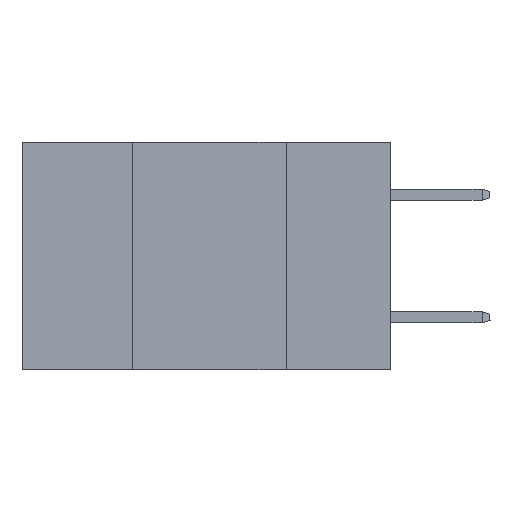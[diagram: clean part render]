
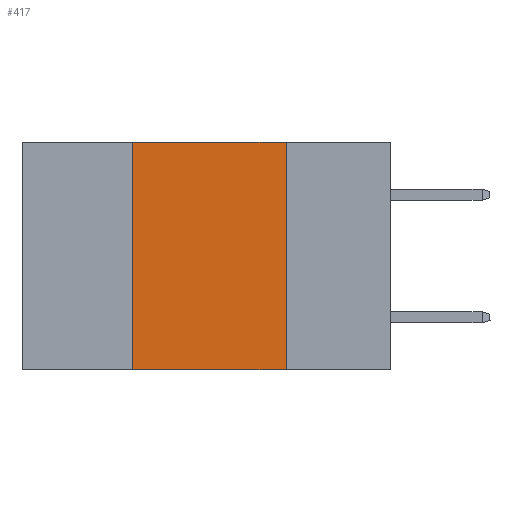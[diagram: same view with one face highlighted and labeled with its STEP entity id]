
A CAD part, left-side view. The second image highlights one B-rep face of the part: STEP entity #417.
In plain terms, the highlighted planar face has unit normal (-1, 0, 0).
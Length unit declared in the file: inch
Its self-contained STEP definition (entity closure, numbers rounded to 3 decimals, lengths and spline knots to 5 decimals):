
#258 = CARTESIAN_POINT ( 'NONE',  ( 0., 0.6, -0.37 ) ) ;
#352 = VERTEX_POINT ( 'NONE', #11496 ) ;
#417 = ADVANCED_FACE ( 'NONE', ( #10884 ), #7326, .F. ) ;
#541 = EDGE_CURVE ( 'NONE', #970, #2907, #6968, .T. ) ;
#970 = VERTEX_POINT ( 'NONE', #1032 ) ;
#1032 = CARTESIAN_POINT ( 'NONE',  ( 0., 0.42, 0. ) ) ;
#1484 = CARTESIAN_POINT ( 'NONE',  ( 0., 0.17, 0. ) ) ;
#1589 = DIRECTION ( 'NONE',  ( 0., 0., -1. ) ) ;
#1726 = VECTOR ( 'NONE', #6818, 39.37008 ) ;
#1944 = EDGE_CURVE ( 'NONE', #2907, #6523, #7515, .T. ) ;
#2330 = ORIENTED_EDGE ( 'NONE', *, *, #8912, .F. ) ;
#2578 = DIRECTION ( 'NONE',  ( 0., -1., 0. ) ) ;
#2799 = EDGE_LOOP ( 'NONE', ( #12917, #10776, #2330, #3035 ) ) ;
#2907 = VERTEX_POINT ( 'NONE', #8770 ) ;
#3035 = ORIENTED_EDGE ( 'NONE', *, *, #3751, .T. ) ;
#3473 = CARTESIAN_POINT ( 'NONE',  ( 0., 0.42, 0. ) ) ;
#3667 = AXIS2_PLACEMENT_3D ( 'NONE', #11255, #7296, #7279 ) ;
#3751 = EDGE_CURVE ( 'NONE', #352, #6523, #13833, .T. ) ;
#4753 = LINE ( 'NONE', #3473, #1726 ) ;
#5833 = DIRECTION ( 'NONE',  ( 0., -1., 0. ) ) ;
#6332 = CARTESIAN_POINT ( 'NONE',  ( 0., 0.6, 0. ) ) ;
#6523 = VERTEX_POINT ( 'NONE', #6580 ) ;
#6580 = CARTESIAN_POINT ( 'NONE',  ( 0., 0.17, -0.37 ) ) ;
#6818 = DIRECTION ( 'NONE',  ( 0., 0., 1. ) ) ;
#6968 = LINE ( 'NONE', #6332, #9509 ) ;
#7279 = DIRECTION ( 'NONE',  ( 0., 0., -1. ) ) ;
#7296 = DIRECTION ( 'NONE',  ( 1., 0., 0. ) ) ;
#7326 = PLANE ( 'NONE',  #3667 ) ;
#7515 = LINE ( 'NONE', #1484, #12547 ) ;
#8770 = CARTESIAN_POINT ( 'NONE',  ( 0., 0.17, 0. ) ) ;
#8912 = EDGE_CURVE ( 'NONE', #352, #970, #4753, .T. ) ;
#9509 = VECTOR ( 'NONE', #5833, 39.37008 ) ;
#10776 = ORIENTED_EDGE ( 'NONE', *, *, #541, .F. ) ;
#10884 = FACE_OUTER_BOUND ( 'NONE', #2799, .T. ) ;
#11029 = VECTOR ( 'NONE', #2578, 39.37008 ) ;
#11255 = CARTESIAN_POINT ( 'NONE',  ( 0., 0.6, 0. ) ) ;
#11496 = CARTESIAN_POINT ( 'NONE',  ( 0., 0.42, -0.37 ) ) ;
#12547 = VECTOR ( 'NONE', #1589, 39.37008 ) ;
#12917 = ORIENTED_EDGE ( 'NONE', *, *, #1944, .F. ) ;
#13833 = LINE ( 'NONE', #258, #11029 ) ;
